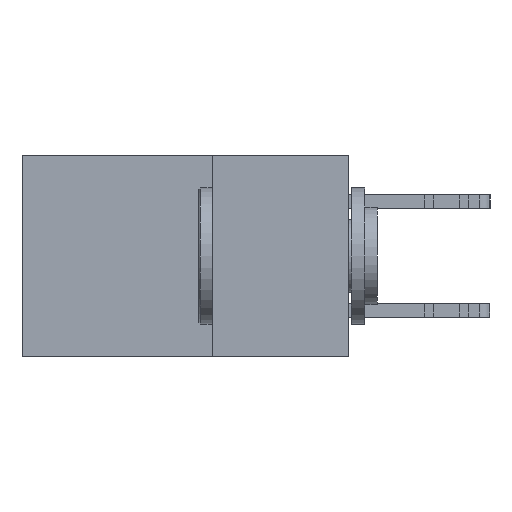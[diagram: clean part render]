
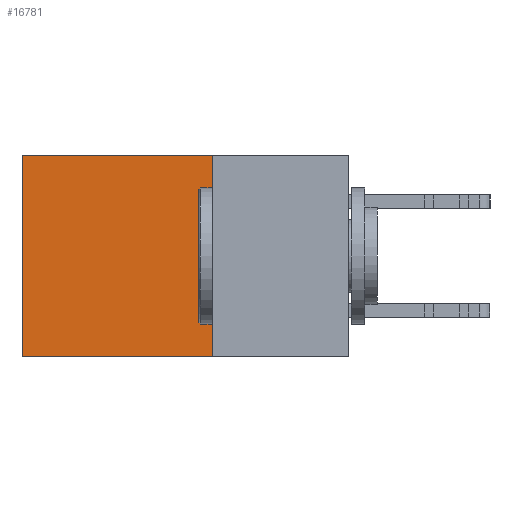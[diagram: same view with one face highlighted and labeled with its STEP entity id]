
A CAD part, left-side view. The second image highlights one B-rep face of the part: STEP entity #16781.
In plain terms, the highlighted planar face has unit normal (-1, 0, 0).
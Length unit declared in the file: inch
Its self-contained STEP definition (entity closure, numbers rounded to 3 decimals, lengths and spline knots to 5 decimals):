
#286 = EDGE_CURVE ( 'NONE', #13977, #31363, #15575, .T. ) ;
#1908 = EDGE_CURVE ( 'NONE', #3780, #31363, #10977, .T. ) ;
#3096 = FACE_OUTER_BOUND ( 'NONE', #11830, .T. ) ;
#3780 = VERTEX_POINT ( 'NONE', #5233 ) ;
#4762 = VECTOR ( 'NONE', #18310, 39.37008 ) ;
#5233 = CARTESIAN_POINT ( 'NONE',  ( 0.298, 0.6, 0. ) ) ;
#8957 = ORIENTED_EDGE ( 'NONE', *, *, #28355, .T. ) ;
#9651 = DIRECTION ( 'NONE',  ( 1., 0., 0. ) ) ;
#9865 = LINE ( 'NONE', #28680, #22983 ) ;
#10658 = CARTESIAN_POINT ( 'NONE',  ( 0.298, 0.25, 0. ) ) ;
#10927 = CARTESIAN_POINT ( 'NONE',  ( 0.298, 0.25, 0. ) ) ;
#10977 = LINE ( 'NONE', #18313, #4762 ) ;
#11830 = EDGE_LOOP ( 'NONE', ( #18567, #32677, #30519, #8957 ) ) ;
#13313 = DIRECTION ( 'NONE',  ( 0., 1., 0. ) ) ;
#13977 = VERTEX_POINT ( 'NONE', #32261 ) ;
#15081 = EDGE_CURVE ( 'NONE', #19582, #13977, #9865, .T. ) ;
#15575 = LINE ( 'NONE', #23202, #20877 ) ;
#15577 = DIRECTION ( 'NONE',  ( 0., 0., -1. ) ) ;
#16781 = ADVANCED_FACE ( 'NONE', ( #3096 ), #25355, .F. ) ;
#18310 = DIRECTION ( 'NONE',  ( 0., 0., -1. ) ) ;
#18313 = CARTESIAN_POINT ( 'NONE',  ( 0.298, 0.6, 0. ) ) ;
#18567 = ORIENTED_EDGE ( 'NONE', *, *, #1908, .T. ) ;
#19582 = VERTEX_POINT ( 'NONE', #10927 ) ;
#20877 = VECTOR ( 'NONE', #22625, 39.37008 ) ;
#22625 = DIRECTION ( 'NONE',  ( 0., 1., 0. ) ) ;
#22983 = VECTOR ( 'NONE', #15577, 39.37008 ) ;
#23150 = VECTOR ( 'NONE', #13313, 39.37008 ) ;
#23202 = CARTESIAN_POINT ( 'NONE',  ( 0.298, 0.25, -0.37 ) ) ;
#25134 = CARTESIAN_POINT ( 'NONE',  ( 0.298, 0.6, -0.37 ) ) ;
#25234 = CARTESIAN_POINT ( 'NONE',  ( 0.298, 0.25, 0. ) ) ;
#25355 = PLANE ( 'NONE',  #28727 ) ;
#27992 = DIRECTION ( 'NONE',  ( 0., 0., -1. ) ) ;
#28355 = EDGE_CURVE ( 'NONE', #19582, #3780, #30866, .T. ) ;
#28680 = CARTESIAN_POINT ( 'NONE',  ( 0.298, 0.25, 0. ) ) ;
#28727 = AXIS2_PLACEMENT_3D ( 'NONE', #25234, #9651, #27992 ) ;
#30519 = ORIENTED_EDGE ( 'NONE', *, *, #15081, .F. ) ;
#30866 = LINE ( 'NONE', #10658, #23150 ) ;
#31363 = VERTEX_POINT ( 'NONE', #25134 ) ;
#32261 = CARTESIAN_POINT ( 'NONE',  ( 0.298, 0.25, -0.37 ) ) ;
#32677 = ORIENTED_EDGE ( 'NONE', *, *, #286, .F. ) ;
